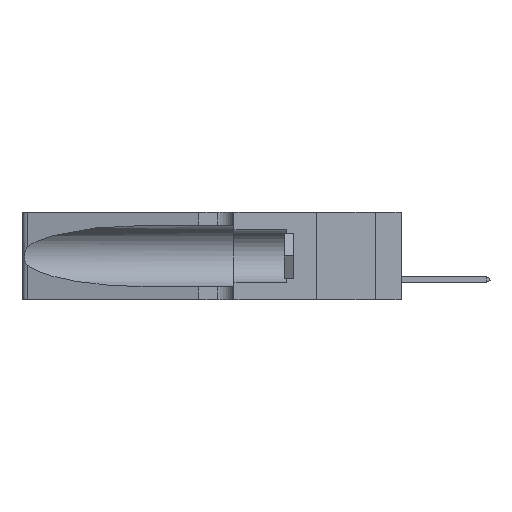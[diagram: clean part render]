
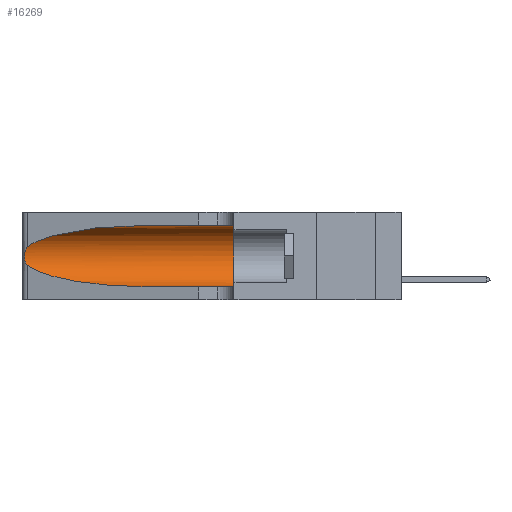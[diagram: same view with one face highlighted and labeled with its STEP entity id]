
A CAD part, left-side view. The second image highlights one B-rep face of the part: STEP entity #16269.
In plain terms, the highlighted cylindrical face has radius 3.308 mm (diameter 6.617 mm), a partial arc.
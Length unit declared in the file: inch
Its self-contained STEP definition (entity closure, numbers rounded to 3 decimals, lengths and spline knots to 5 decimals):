
#588 = VERTEX_POINT ( 'NONE', #10816 ) ;
#1172 = CARTESIAN_POINT ( 'NONE',  ( 0.1305, 0.35, 0.31525 ) ) ;
#1802 = CARTESIAN_POINT ( 'NONE',  ( 0.25487, 1.22718, 0.14631 ) ) ;
#2156 = CARTESIAN_POINT ( 'NONE',  ( 0.25787, 1.23484, 0.2124 ) ) ;
#2408 = CARTESIAN_POINT ( 'NONE',  ( 0.25639, 1.23184, 0.21858 ) ) ;
#2804 = CARTESIAN_POINT ( 'NONE',  ( 0.18966, 0.96281, 0.05475 ) ) ;
#3604 = DIRECTION ( 'NONE',  ( 0., -1., 0. ) ) ;
#3848 = DIRECTION ( 'NONE',  ( 0., -1., 0. ) ) ;
#4060 = EDGE_CURVE ( 'NONE', #4354, #4735, #34708, .T. ) ;
#4354 = VERTEX_POINT ( 'NONE', #20085 ) ;
#4735 = VERTEX_POINT ( 'NONE', #1172 ) ;
#5241 = EDGE_LOOP ( 'NONE', ( #15234, #23120, #15159, #30108, #29636, #9452 ) ) ;
#5256 = CARTESIAN_POINT ( 'NONE',  ( 0.26075, 1.23896, 0.19203 ) ) ;
#5632 = CARTESIAN_POINT ( 'NONE',  ( 0.25856, 1.23593, 0.16098 ) ) ;
#6133 = DIRECTION ( 'NONE',  ( 0., -1., 0. ) ) ;
#7441 = EDGE_CURVE ( 'NONE', #4735, #18809, #10401, .T. ) ;
#8402 =( BOUNDED_CURVE ( )  B_SPLINE_CURVE ( 3, ( #14141, #17225, #25727, #20186 ),
 .UNSPECIFIED., .F., .T. ) 
 B_SPLINE_CURVE_WITH_KNOTS ( ( 4, 4 ),
 ( 1.5708, 2.84003 ),
 .UNSPECIFIED. ) 
 CURVE ( )  GEOMETRIC_REPRESENTATION_ITEM ( )  RATIONAL_B_SPLINE_CURVE ( ( 1., 0.87, 0.87, 1. ) ) 
 REPRESENTATION_ITEM ( '' )  );
#8506 = CARTESIAN_POINT ( 'NONE',  ( 0.26018, 1.23835, 0.19895 ) ) ;
#9452 = ORIENTED_EDGE ( 'NONE', *, *, #4060, .F. ) ;
#9476 = VECTOR ( 'NONE', #3604, 39.37008 ) ;
#9697 = CARTESIAN_POINT ( 'NONE',  ( 0.1305, 1.61858, 0.185 ) ) ;
#10168 = DIRECTION ( 'NONE',  ( 0., 1., 0. ) ) ;
#10282 = CARTESIAN_POINT ( 'NONE',  ( 0.25555, 1.22994, 0.2215 ) ) ;
#10401 = CIRCLE ( 'NONE', #25906, 0.13025 ) ;
#10561 = CARTESIAN_POINT ( 'NONE',  ( 0.25487, 1.22718, 0.22369 ) ) ;
#10816 = CARTESIAN_POINT ( 'NONE',  ( 0.25487, 1.22718, 0.14631 ) ) ;
#11267 = FACE_OUTER_BOUND ( 'NONE', #5241, .T. ) ;
#13924 = CARTESIAN_POINT ( 'NONE',  ( 0.25854, 1.2359, 0.20912 ) ) ;
#14012 = VERTEX_POINT ( 'NONE', #33176 ) ;
#14141 = CARTESIAN_POINT ( 'NONE',  ( 0.1305, 0.72297, 0.31525 ) ) ;
#14304 = CARTESIAN_POINT ( 'NONE',  ( 0.26075, 1.23896, 0.178 ) ) ;
#14716 = EDGE_CURVE ( 'NONE', #4354, #35055, #8402, .T. ) ;
#15159 = ORIENTED_EDGE ( 'NONE', *, *, #33298, .T. ) ;
#15234 = ORIENTED_EDGE ( 'NONE', *, *, #14716, .T. ) ;
#15833 = CYLINDRICAL_SURFACE ( 'NONE', #17927, 0.13025 ) ;
#15866 = DIRECTION ( 'NONE',  ( 0., 0., -1. ) ) ;
#16269 = ADVANCED_FACE ( 'NONE', ( #11267 ), #15833, .F. ) ;
#17225 = CARTESIAN_POINT ( 'NONE',  ( 0.18966, 0.96281, 0.31525 ) ) ;
#17375 = LINE ( 'NONE', #33190, #9476 ) ;
#17927 = AXIS2_PLACEMENT_3D ( 'NONE', #9697, #3848, #15866 ) ;
#18809 = VERTEX_POINT ( 'NONE', #25830 ) ;
#19799 = CARTESIAN_POINT ( 'NONE',  ( 0.25487, 1.22718, 0.22369 ) ) ;
#20085 = CARTESIAN_POINT ( 'NONE',  ( 0.1305, 0.72297, 0.31525 ) ) ;
#20154 = EDGE_CURVE ( 'NONE', #14012, #18809, #17375, .T. ) ;
#20186 = CARTESIAN_POINT ( 'NONE',  ( 0.25487, 1.22718, 0.22369 ) ) ;
#23120 = ORIENTED_EDGE ( 'NONE', *, *, #30983, .T. ) ;
#23327 = CARTESIAN_POINT ( 'NONE',  ( 0.26017, 1.23833, 0.17102 ) ) ;
#25727 = CARTESIAN_POINT ( 'NONE',  ( 0.2373, 1.15595, 0.28018 ) ) ;
#25830 = CARTESIAN_POINT ( 'NONE',  ( 0.1305, 0.35, 0.05475 ) ) ;
#25892 = CARTESIAN_POINT ( 'NONE',  ( 0.25789, 1.23486, 0.15765 ) ) ;
#25906 = AXIS2_PLACEMENT_3D ( 'NONE', #27835, #10168, #30844 ) ;
#27835 = CARTESIAN_POINT ( 'NONE',  ( 0.1305, 0.35, 0.185 ) ) ;
#28271 =( BOUNDED_CURVE ( )  B_SPLINE_CURVE ( 3, ( #1802, #37467, #2804, #34885 ),
 .UNSPECIFIED., .F., .F. ) 
 B_SPLINE_CURVE_WITH_KNOTS ( ( 4, 4 ),
 ( 3.44316, 4.71239 ),
 .UNSPECIFIED. ) 
 CURVE ( )  GEOMETRIC_REPRESENTATION_ITEM ( )  RATIONAL_B_SPLINE_CURVE ( ( 1., 0.87, 0.87, 1. ) ) 
 REPRESENTATION_ITEM ( '' )  );
#29636 = ORIENTED_EDGE ( 'NONE', *, *, #7441, .F. ) ;
#30108 = ORIENTED_EDGE ( 'NONE', *, *, #20154, .T. ) ;
#30844 = DIRECTION ( 'NONE',  ( 0., 0., 1. ) ) ;
#30983 = EDGE_CURVE ( 'NONE', #35055, #588, #37012, .T. ) ;
#33176 = CARTESIAN_POINT ( 'NONE',  ( 0.1305, 0.72297, 0.05475 ) ) ;
#33190 = CARTESIAN_POINT ( 'NONE',  ( 0.1305, 1.61858, 0.05475 ) ) ;
#33298 = EDGE_CURVE ( 'NONE', #588, #14012, #28271, .T. ) ;
#33732 = VECTOR ( 'NONE', #6133, 39.37008 ) ;
#34708 = LINE ( 'NONE', #35611, #33732 ) ;
#34885 = CARTESIAN_POINT ( 'NONE',  ( 0.1305, 0.72297, 0.05475 ) ) ;
#34983 = CARTESIAN_POINT ( 'NONE',  ( 0.25487, 1.22718, 0.14631 ) ) ;
#35055 = VERTEX_POINT ( 'NONE', #19799 ) ;
#35611 = CARTESIAN_POINT ( 'NONE',  ( 0.1305, 1.61858, 0.31525 ) ) ;
#37012 = B_SPLINE_CURVE_WITH_KNOTS ( 'NONE', 3,
 ( #10561, #10282, #2408, #2156, #13924, #8506, #5256, #14304, #23327, #5632, #25892, #37808, #37938, #34983 ),
 .UNSPECIFIED., .F., .F.,
 ( 4, 2, 2, 2, 2, 2, 4 ),
 ( 0., 0.00027, 0.00053, 0.00107, 0.0016, 0.00187, 0.00214 ),
 .UNSPECIFIED. ) ;
#37467 = CARTESIAN_POINT ( 'NONE',  ( 0.2373, 1.15595, 0.08982 ) ) ;
#37808 = CARTESIAN_POINT ( 'NONE',  ( 0.25639, 1.23186, 0.15144 ) ) ;
#37938 = CARTESIAN_POINT ( 'NONE',  ( 0.25555, 1.22993, 0.14849 ) ) ;
